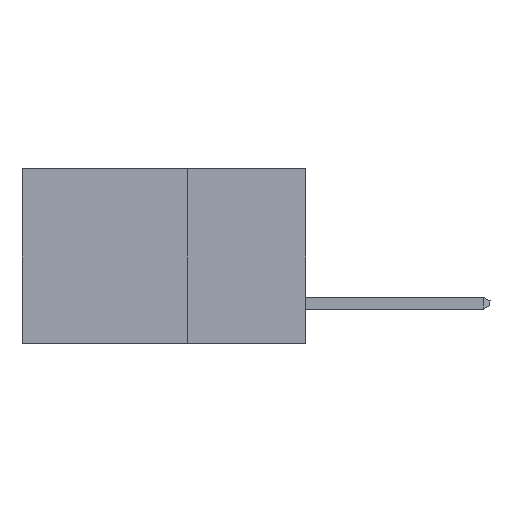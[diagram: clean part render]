
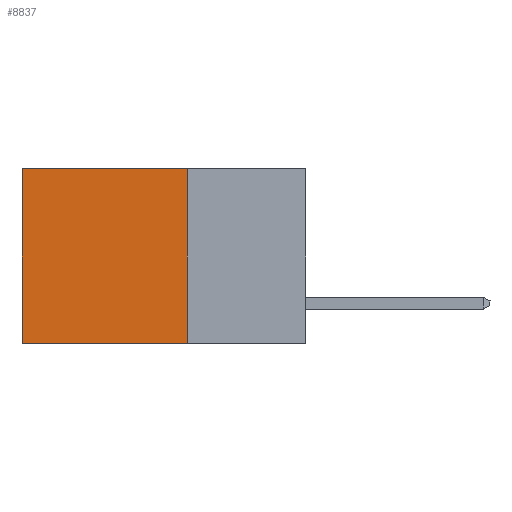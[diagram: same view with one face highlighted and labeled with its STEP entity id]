
A CAD part, left-side view. The second image highlights one B-rep face of the part: STEP entity #8837.
In plain terms, the highlighted planar face has unit normal (-1, 0, 0).
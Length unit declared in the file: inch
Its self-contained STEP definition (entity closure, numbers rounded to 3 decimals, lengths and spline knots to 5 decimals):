
#341 = FACE_OUTER_BOUND ( 'NONE', #7616, .T. ) ;
#473 = VERTEX_POINT ( 'NONE', #6031 ) ;
#1483 = VECTOR ( 'NONE', #2869, 39.37008 ) ;
#1592 = DIRECTION ( 'NONE',  ( 1., 0., 0. ) ) ;
#1633 = CARTESIAN_POINT ( 'NONE',  ( 0.2615, 0.25, -0.37 ) ) ;
#1955 = ORIENTED_EDGE ( 'NONE', *, *, #3086, .T. ) ;
#2129 = DIRECTION ( 'NONE',  ( 0., 0., -1. ) ) ;
#2741 = EDGE_CURVE ( 'NONE', #11558, #473, #14490, .T. ) ;
#2869 = DIRECTION ( 'NONE',  ( 0., 0., -1. ) ) ;
#3086 = EDGE_CURVE ( 'NONE', #11558, #6604, #7566, .T. ) ;
#3141 = ORIENTED_EDGE ( 'NONE', *, *, #4477, .F. ) ;
#3791 = PLANE ( 'NONE',  #10018 ) ;
#4236 = VERTEX_POINT ( 'NONE', #9637 ) ;
#4477 = EDGE_CURVE ( 'NONE', #473, #4236, #6836, .T. ) ;
#5727 = CARTESIAN_POINT ( 'NONE',  ( 0.2615, 0.25, -0.37 ) ) ;
#5993 = EDGE_CURVE ( 'NONE', #6604, #4236, #7064, .T. ) ;
#6031 = CARTESIAN_POINT ( 'NONE',  ( 0.2615, 0.25, -0.37 ) ) ;
#6138 = DIRECTION ( 'NONE',  ( 0., 0., -1. ) ) ;
#6604 = VERTEX_POINT ( 'NONE', #8539 ) ;
#6836 = LINE ( 'NONE', #5727, #12533 ) ;
#7064 = LINE ( 'NONE', #10500, #8485 ) ;
#7566 = LINE ( 'NONE', #12030, #13509 ) ;
#7616 = EDGE_LOOP ( 'NONE', ( #13100, #3141, #10206, #1955 ) ) ;
#7816 = DIRECTION ( 'NONE',  ( 0., 1., 0. ) ) ;
#8485 = VECTOR ( 'NONE', #2129, 39.37008 ) ;
#8539 = CARTESIAN_POINT ( 'NONE',  ( 0.2615, 0.6, 0. ) ) ;
#8837 = ADVANCED_FACE ( 'NONE', ( #341 ), #3791, .F. ) ;
#9637 = CARTESIAN_POINT ( 'NONE',  ( 0.2615, 0.6, -0.37 ) ) ;
#9649 = DIRECTION ( 'NONE',  ( 0., 1., 0. ) ) ;
#10018 = AXIS2_PLACEMENT_3D ( 'NONE', #11781, #1592, #6138 ) ;
#10206 = ORIENTED_EDGE ( 'NONE', *, *, #2741, .F. ) ;
#10500 = CARTESIAN_POINT ( 'NONE',  ( 0.2615, 0.6, -0.37 ) ) ;
#11558 = VERTEX_POINT ( 'NONE', #12888 ) ;
#11781 = CARTESIAN_POINT ( 'NONE',  ( 0.2615, 0.25, -0.37 ) ) ;
#12030 = CARTESIAN_POINT ( 'NONE',  ( 0.2615, 0.25, 0. ) ) ;
#12533 = VECTOR ( 'NONE', #7816, 39.37008 ) ;
#12888 = CARTESIAN_POINT ( 'NONE',  ( 0.2615, 0.25, 0. ) ) ;
#13100 = ORIENTED_EDGE ( 'NONE', *, *, #5993, .T. ) ;
#13509 = VECTOR ( 'NONE', #9649, 39.37008 ) ;
#14490 = LINE ( 'NONE', #1633, #1483 ) ;
